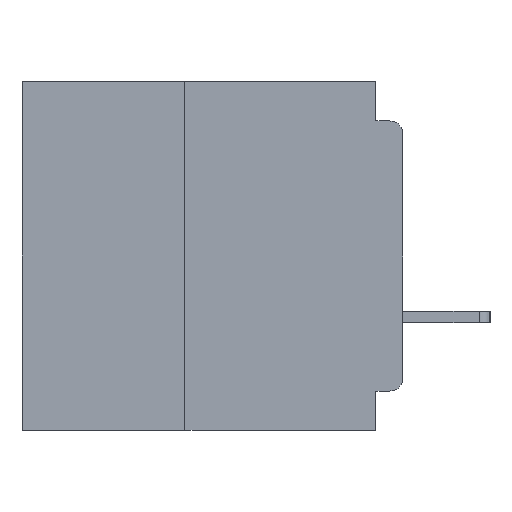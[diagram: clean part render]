
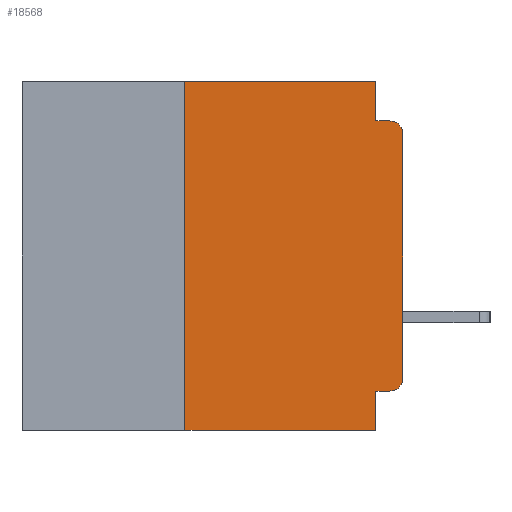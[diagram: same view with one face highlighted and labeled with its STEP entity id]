
A CAD part, left-side view. The second image highlights one B-rep face of the part: STEP entity #18568.
In plain terms, the highlighted planar face has unit normal (-1, 0, 0).
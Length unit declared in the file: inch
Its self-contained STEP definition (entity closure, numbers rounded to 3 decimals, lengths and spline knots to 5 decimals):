
#2263 = CARTESIAN_POINT ( 'NONE',  ( 0., 0.25, -0.4 ) ) ;
#2297 = EDGE_CURVE ( 'NONE', #10984, #27576, #52450, .T. ) ;
#2732 = CARTESIAN_POINT ( 'NONE',  ( 0., 0.031, -0.4 ) ) ;
#4156 = CARTESIAN_POINT ( 'NONE',  ( 0., 0., -0.34 ) ) ;
#4537 = DIRECTION ( 'NONE',  ( 0., -1., 0. ) ) ;
#5939 = CARTESIAN_POINT ( 'NONE',  ( 0., 0.015, -0.06 ) ) ;
#6275 = ORIENTED_EDGE ( 'NONE', *, *, #18035, .T. ) ;
#6484 = EDGE_CURVE ( 'NONE', #10984, #43859, #21243, .T. ) ;
#6571 = CARTESIAN_POINT ( 'NONE',  ( 0., 0.437, -0.4 ) ) ;
#7187 = VECTOR ( 'NONE', #27319, 39.37008 ) ;
#7824 = CARTESIAN_POINT ( 'NONE',  ( 0., 0.015, -0.34 ) ) ;
#7974 = EDGE_CURVE ( 'NONE', #8647, #14977, #14617, .T. ) ;
#8647 = VERTEX_POINT ( 'NONE', #4156 ) ;
#9829 = LINE ( 'NONE', #2732, #12463 ) ;
#10150 = VECTOR ( 'NONE', #32449, 39.37008 ) ;
#10162 = DIRECTION ( 'NONE',  ( 0., 0., -1. ) ) ;
#10491 = ORIENTED_EDGE ( 'NONE', *, *, #2297, .T. ) ;
#10984 = VERTEX_POINT ( 'NONE', #2263 ) ;
#11254 = CARTESIAN_POINT ( 'NONE',  ( 0., 0.015, -0.045 ) ) ;
#12048 = DIRECTION ( 'NONE',  ( 0., 0., -1. ) ) ;
#12189 = CARTESIAN_POINT ( 'NONE',  ( 0., 0.437, 0. ) ) ;
#12463 = VECTOR ( 'NONE', #31936, 39.37008 ) ;
#13185 = VECTOR ( 'NONE', #18066, 39.37008 ) ;
#13432 = EDGE_CURVE ( 'NONE', #19641, #27445, #53339, .T. ) ;
#14457 = LINE ( 'NONE', #41607, #35143 ) ;
#14617 = LINE ( 'NONE', #37182, #39188 ) ;
#14782 = VERTEX_POINT ( 'NONE', #52816 ) ;
#14977 = VERTEX_POINT ( 'NONE', #33413 ) ;
#15107 = EDGE_CURVE ( 'NONE', #14782, #30012, #36492, .T. ) ;
#15544 = ORIENTED_EDGE ( 'NONE', *, *, #15107, .F. ) ;
#18035 = EDGE_CURVE ( 'NONE', #14782, #8647, #24603, .T. ) ;
#18066 = DIRECTION ( 'NONE',  ( 0., 1., 0. ) ) ;
#18568 = ADVANCED_FACE ( 'NONE', ( #20653 ), #36993, .F. ) ;
#18891 = CARTESIAN_POINT ( 'NONE',  ( 0., 0.437, 0. ) ) ;
#19449 = ORIENTED_EDGE ( 'NONE', *, *, #6484, .F. ) ;
#19641 = VERTEX_POINT ( 'NONE', #37742 ) ;
#20262 = AXIS2_PLACEMENT_3D ( 'NONE', #7824, #36864, #12048 ) ;
#20429 = CARTESIAN_POINT ( 'NONE',  ( 0., 0.031, -0.355 ) ) ;
#20554 = DIRECTION ( 'NONE',  ( 0., 0., -1. ) ) ;
#20653 = FACE_OUTER_BOUND ( 'NONE', #52999, .T. ) ;
#21243 = LINE ( 'NONE', #48793, #10150 ) ;
#22330 = ORIENTED_EDGE ( 'NONE', *, *, #44388, .T. ) ;
#22508 = EDGE_CURVE ( 'NONE', #27445, #37166, #14457, .T. ) ;
#22573 = ORIENTED_EDGE ( 'NONE', *, *, #26250, .F. ) ;
#22921 = CARTESIAN_POINT ( 'NONE',  ( 0., 0.031, 0. ) ) ;
#23020 = DIRECTION ( 'NONE',  ( 0., -1., 0. ) ) ;
#23931 = CARTESIAN_POINT ( 'NONE',  ( 0., 0.25, 0. ) ) ;
#24603 = CIRCLE ( 'NONE', #20262, 0.015 ) ;
#25332 = CARTESIAN_POINT ( 'NONE',  ( 0., 0.031, -0.4 ) ) ;
#26045 = ORIENTED_EDGE ( 'NONE', *, *, #46840, .F. ) ;
#26250 = EDGE_CURVE ( 'NONE', #30012, #27576, #9829, .T. ) ;
#27319 = DIRECTION ( 'NONE',  ( 0., -1., 0. ) ) ;
#27445 = VERTEX_POINT ( 'NONE', #39413 ) ;
#27576 = VERTEX_POINT ( 'NONE', #25332 ) ;
#27873 = ORIENTED_EDGE ( 'NONE', *, *, #22508, .F. ) ;
#29278 = AXIS2_PLACEMENT_3D ( 'NONE', #12189, #45265, #20554 ) ;
#30012 = VERTEX_POINT ( 'NONE', #20429 ) ;
#31063 = DIRECTION ( 'NONE',  ( 0., 0., -1. ) ) ;
#31936 = DIRECTION ( 'NONE',  ( 0., 0., -1. ) ) ;
#32449 = DIRECTION ( 'NONE',  ( 0., 0., 1. ) ) ;
#33413 = CARTESIAN_POINT ( 'NONE',  ( 0., 0., -0.06 ) ) ;
#34494 = CARTESIAN_POINT ( 'NONE',  ( 0., 0., -0.355 ) ) ;
#34807 = ORIENTED_EDGE ( 'NONE', *, *, #7974, .T. ) ;
#34892 = AXIS2_PLACEMENT_3D ( 'NONE', #5939, #34998, #10162 ) ;
#34998 = DIRECTION ( 'NONE',  ( -1., 0., 0. ) ) ;
#35143 = VECTOR ( 'NONE', #4537, 39.37008 ) ;
#36492 = LINE ( 'NONE', #34494, #13185 ) ;
#36864 = DIRECTION ( 'NONE',  ( -1., 0., 0. ) ) ;
#36993 = PLANE ( 'NONE',  #29278 ) ;
#37166 = VERTEX_POINT ( 'NONE', #11254 ) ;
#37182 = CARTESIAN_POINT ( 'NONE',  ( 0., 0., 0. ) ) ;
#37632 = VECTOR ( 'NONE', #23020, 39.37008 ) ;
#37742 = CARTESIAN_POINT ( 'NONE',  ( 0., 0.031, 0. ) ) ;
#38930 = LINE ( 'NONE', #18891, #37632 ) ;
#39188 = VECTOR ( 'NONE', #41312, 39.37008 ) ;
#39413 = CARTESIAN_POINT ( 'NONE',  ( 0., 0.031, -0.045 ) ) ;
#41312 = DIRECTION ( 'NONE',  ( 0., 0., 1. ) ) ;
#41607 = CARTESIAN_POINT ( 'NONE',  ( 0., 0., -0.045 ) ) ;
#42479 = VECTOR ( 'NONE', #31063, 39.37008 ) ;
#43859 = VERTEX_POINT ( 'NONE', #23931 ) ;
#44388 = EDGE_CURVE ( 'NONE', #14977, #37166, #46839, .T. ) ;
#45265 = DIRECTION ( 'NONE',  ( 1., 0., 0. ) ) ;
#46839 = CIRCLE ( 'NONE', #34892, 0.015 ) ;
#46840 = EDGE_CURVE ( 'NONE', #43859, #19641, #38930, .T. ) ;
#48793 = CARTESIAN_POINT ( 'NONE',  ( 0., 0.25, -0.4 ) ) ;
#52369 = ORIENTED_EDGE ( 'NONE', *, *, #13432, .F. ) ;
#52450 = LINE ( 'NONE', #6571, #7187 ) ;
#52816 = CARTESIAN_POINT ( 'NONE',  ( 0., 0.015, -0.355 ) ) ;
#52999 = EDGE_LOOP ( 'NONE', ( #34807, #22330, #27873, #52369, #26045, #19449, #10491, #22573, #15544, #6275 ) ) ;
#53339 = LINE ( 'NONE', #22921, #42479 ) ;
